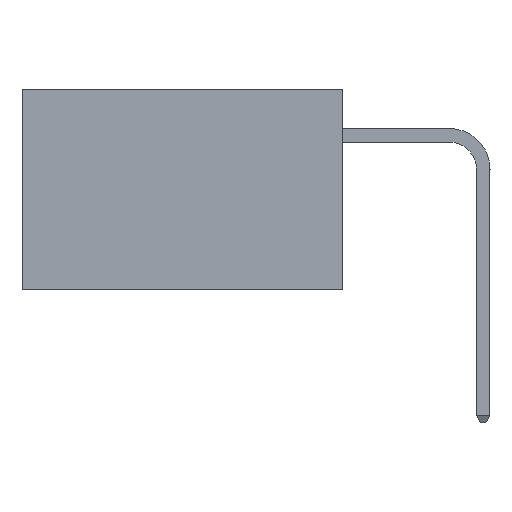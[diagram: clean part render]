
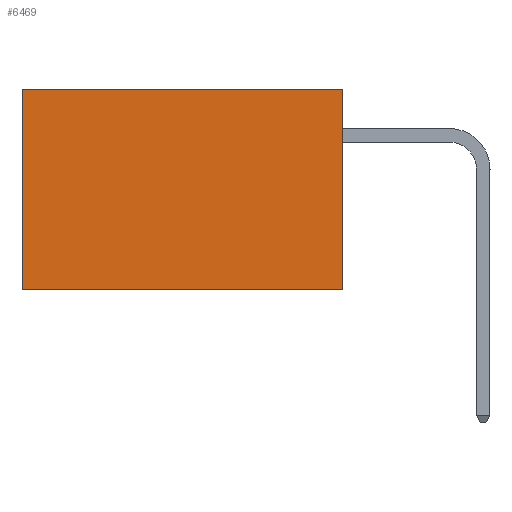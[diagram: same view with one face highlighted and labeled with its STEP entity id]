
A CAD part, left-side view. The second image highlights one B-rep face of the part: STEP entity #6469.
In plain terms, the highlighted planar face has unit normal (-1, 0, 0).
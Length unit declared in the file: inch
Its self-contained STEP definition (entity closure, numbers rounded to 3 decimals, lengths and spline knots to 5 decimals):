
#1683 = FACE_OUTER_BOUND ( 'NONE', #9270, .T. ) ;
#1721 = ORIENTED_EDGE ( 'NONE', *, *, #9557, .F. ) ;
#2086 = LINE ( 'NONE', #3307, #7377 ) ;
#2307 = VECTOR ( 'NONE', #5707, 39.37008 ) ;
#2722 = CARTESIAN_POINT ( 'NONE',  ( 0.277, 0.59, -0.37 ) ) ;
#2917 = LINE ( 'NONE', #5667, #2307 ) ;
#3019 = CARTESIAN_POINT ( 'NONE',  ( 0.277, 0., 0. ) ) ;
#3307 = CARTESIAN_POINT ( 'NONE',  ( 0.277, 0.59, -0.37 ) ) ;
#3411 = CARTESIAN_POINT ( 'NONE',  ( 0.277, 0., 0. ) ) ;
#4321 = DIRECTION ( 'NONE',  ( 0., 0., -1. ) ) ;
#4328 = AXIS2_PLACEMENT_3D ( 'NONE', #7315, #7519, #7210 ) ;
#4682 = DIRECTION ( 'NONE',  ( 0., 1., 0. ) ) ;
#5457 = VECTOR ( 'NONE', #4682, 39.37008 ) ;
#5490 = VERTEX_POINT ( 'NONE', #8581 ) ;
#5667 = CARTESIAN_POINT ( 'NONE',  ( 0.277, 0., -0.37 ) ) ;
#5707 = DIRECTION ( 'NONE',  ( 0., 0., -1. ) ) ;
#6457 = CARTESIAN_POINT ( 'NONE',  ( 0.277, 0., -0.37 ) ) ;
#6469 = ADVANCED_FACE ( 'NONE', ( #1683 ), #7280, .F. ) ;
#7210 = DIRECTION ( 'NONE',  ( 0., 0., -1. ) ) ;
#7267 = EDGE_CURVE ( 'NONE', #9709, #5490, #7761, .T. ) ;
#7280 = PLANE ( 'NONE',  #4328 ) ;
#7315 = CARTESIAN_POINT ( 'NONE',  ( 0.277, 0., -0.37 ) ) ;
#7377 = VECTOR ( 'NONE', #4321, 39.37008 ) ;
#7423 = LINE ( 'NONE', #11423, #9751 ) ;
#7519 = DIRECTION ( 'NONE',  ( 1., 0., 0. ) ) ;
#7663 = VERTEX_POINT ( 'NONE', #6457 ) ;
#7761 = LINE ( 'NONE', #3411, #5457 ) ;
#8581 = CARTESIAN_POINT ( 'NONE',  ( 0.277, 0.59, 0. ) ) ;
#9270 = EDGE_LOOP ( 'NONE', ( #9378, #1721, #9975, #12530 ) ) ;
#9362 = EDGE_CURVE ( 'NONE', #9709, #7663, #2917, .T. ) ;
#9378 = ORIENTED_EDGE ( 'NONE', *, *, #12033, .T. ) ;
#9557 = EDGE_CURVE ( 'NONE', #7663, #10889, #7423, .T. ) ;
#9709 = VERTEX_POINT ( 'NONE', #3019 ) ;
#9751 = VECTOR ( 'NONE', #11736, 39.37008 ) ;
#9975 = ORIENTED_EDGE ( 'NONE', *, *, #9362, .F. ) ;
#10889 = VERTEX_POINT ( 'NONE', #2722 ) ;
#11423 = CARTESIAN_POINT ( 'NONE',  ( 0.277, 0., -0.37 ) ) ;
#11736 = DIRECTION ( 'NONE',  ( 0., 1., 0. ) ) ;
#12033 = EDGE_CURVE ( 'NONE', #5490, #10889, #2086, .T. ) ;
#12530 = ORIENTED_EDGE ( 'NONE', *, *, #7267, .T. ) ;
